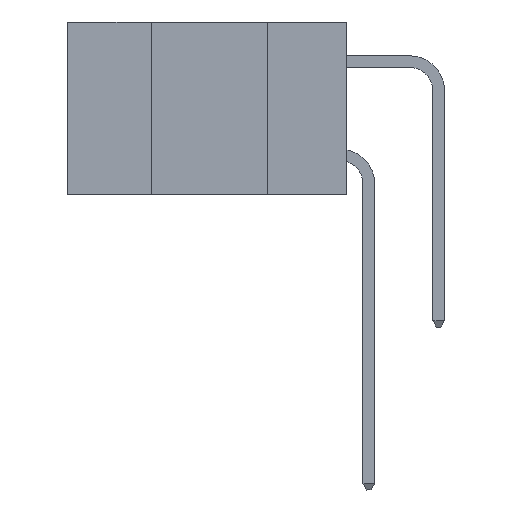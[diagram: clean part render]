
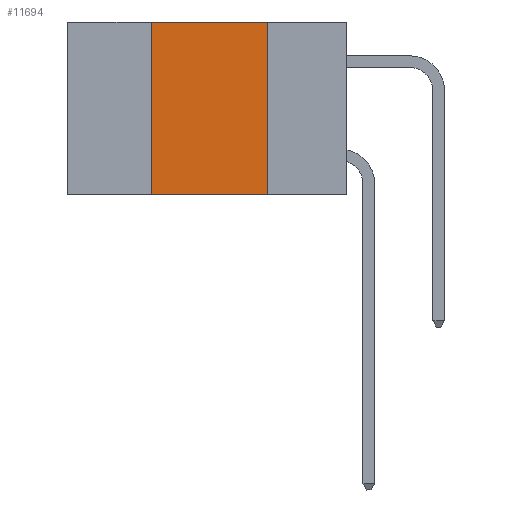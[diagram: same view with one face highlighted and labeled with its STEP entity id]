
A CAD part, left-side view. The second image highlights one B-rep face of the part: STEP entity #11694.
In plain terms, the highlighted planar face has unit normal (-1, 0, 0).
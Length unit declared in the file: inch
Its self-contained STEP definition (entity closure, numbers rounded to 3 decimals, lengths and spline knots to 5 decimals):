
#2137 = VECTOR ( 'NONE', #4995, 39.37008 ) ;
#3927 = ORIENTED_EDGE ( 'NONE', *, *, #4963, .T. ) ;
#3957 = VECTOR ( 'NONE', #5713, 39.37008 ) ;
#4568 = FACE_OUTER_BOUND ( 'NONE', #15846, .T. ) ;
#4963 = EDGE_CURVE ( 'NONE', #11099, #6029, #6774, .T. ) ;
#4995 = DIRECTION ( 'NONE',  ( 0., 0., -1. ) ) ;
#5713 = DIRECTION ( 'NONE',  ( 0., -1., 0. ) ) ;
#6029 = VERTEX_POINT ( 'NONE', #21799 ) ;
#6774 = LINE ( 'NONE', #14448, #21391 ) ;
#7250 = LINE ( 'NONE', #12565, #2137 ) ;
#9268 = CARTESIAN_POINT ( 'NONE',  ( 0., 0.42, 0. ) ) ;
#9308 = CARTESIAN_POINT ( 'NONE',  ( 0., 0.42, 0. ) ) ;
#9801 = CARTESIAN_POINT ( 'NONE',  ( 0., 0.17, 0. ) ) ;
#11099 = VERTEX_POINT ( 'NONE', #18777 ) ;
#11188 = DIRECTION ( 'NONE',  ( 1., 0., 0. ) ) ;
#11694 = ADVANCED_FACE ( 'NONE', ( #4568 ), #13044, .F. ) ;
#11760 = EDGE_CURVE ( 'NONE', #17105, #17255, #13519, .T. ) ;
#12565 = CARTESIAN_POINT ( 'NONE',  ( 0., 0.17, 0. ) ) ;
#13044 = PLANE ( 'NONE',  #22728 ) ;
#13519 = LINE ( 'NONE', #17145, #3957 ) ;
#14247 = LINE ( 'NONE', #9268, #18721 ) ;
#14448 = CARTESIAN_POINT ( 'NONE',  ( 0., 0.6, -0.37 ) ) ;
#15846 = EDGE_LOOP ( 'NONE', ( #24472, #20665, #21847, #3927 ) ) ;
#17105 = VERTEX_POINT ( 'NONE', #9308 ) ;
#17145 = CARTESIAN_POINT ( 'NONE',  ( 0., 0.6, 0. ) ) ;
#17255 = VERTEX_POINT ( 'NONE', #9801 ) ;
#18721 = VECTOR ( 'NONE', #20825, 39.37008 ) ;
#18777 = CARTESIAN_POINT ( 'NONE',  ( 0., 0.42, -0.37 ) ) ;
#20225 = EDGE_CURVE ( 'NONE', #11099, #17105, #14247, .T. ) ;
#20665 = ORIENTED_EDGE ( 'NONE', *, *, #11760, .F. ) ;
#20825 = DIRECTION ( 'NONE',  ( 0., 0., 1. ) ) ;
#21391 = VECTOR ( 'NONE', #22004, 39.37008 ) ;
#21799 = CARTESIAN_POINT ( 'NONE',  ( 0., 0.17, -0.37 ) ) ;
#21847 = ORIENTED_EDGE ( 'NONE', *, *, #20225, .F. ) ;
#22004 = DIRECTION ( 'NONE',  ( 0., -1., 0. ) ) ;
#22267 = EDGE_CURVE ( 'NONE', #17255, #6029, #7250, .T. ) ;
#22620 = CARTESIAN_POINT ( 'NONE',  ( 0., 0.6, 0. ) ) ;
#22728 = AXIS2_PLACEMENT_3D ( 'NONE', #22620, #11188, #24511 ) ;
#24472 = ORIENTED_EDGE ( 'NONE', *, *, #22267, .F. ) ;
#24511 = DIRECTION ( 'NONE',  ( 0., 0., -1. ) ) ;
